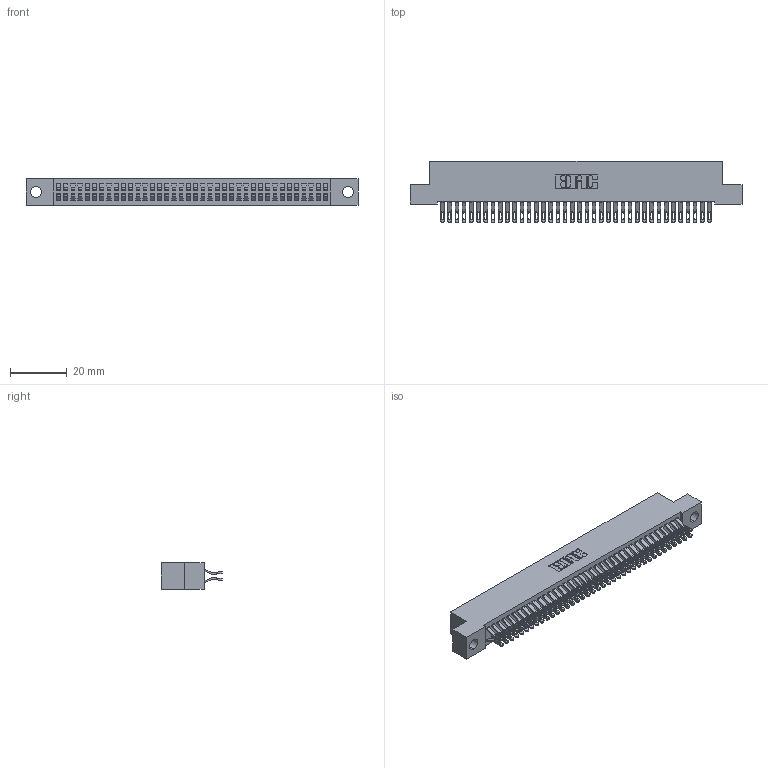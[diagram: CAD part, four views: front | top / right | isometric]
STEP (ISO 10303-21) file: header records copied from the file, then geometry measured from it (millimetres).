
FILE_DESCRIPTION (( 'STEP AP203' ), '1' );
FILE_NAME ('392-076-555-204.STEP', '2019-10-09T13:37:50', ( '' ), ( '' ), 'SwSTEP 2.0', 'SolidWorks 2016', '' );
FILE_SCHEMA (( 'CONFIG_CONTROL_DESIGN' ));
Length unit declared in the file: inch
Products named in the file (3): 342 Part_.156 TH; 345-292-001_555 Tail; 392-076-555-204
Assembly tree (77 placements, depth 2):
  392-076-555-204
    342 Part_.156 TH
    345-292-001_555 Tail  x76
Bounding box: 116.84 x 21.47 x 9.4 mm (x, y, z)
Volume: 10603.3 mm3; surface area: 17720.5 mm2
Topology: 77 solids, 77 shells, 4518 faces, 14207 edges, 9470 vertices
Faces by surface type: plane 2650, cylinder 1868
Entity records: 25161 total; most frequent: CARTESIAN_POINT 4208, ORIENTED_EDGE 4114, DIRECTION 3573, EDGE_CURVE 2057, VECTOR 1909, LINE 1909, VERTEX_POINT 1370, AXIS2_PLACEMENT_3D 832
